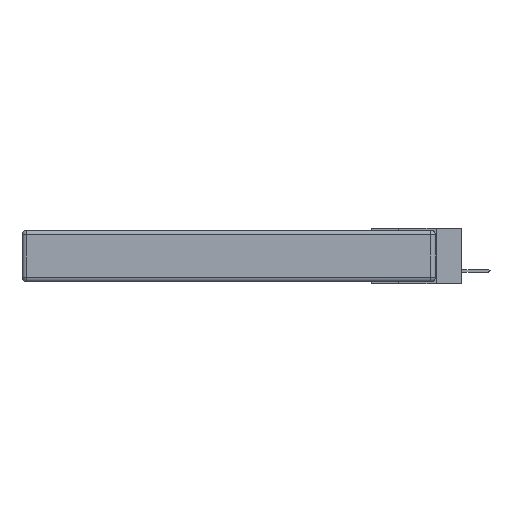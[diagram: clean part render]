
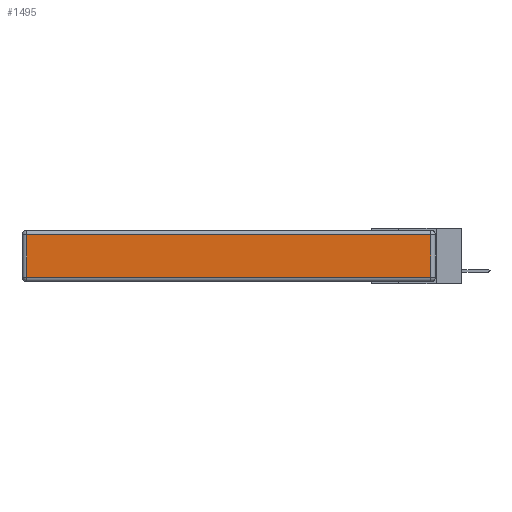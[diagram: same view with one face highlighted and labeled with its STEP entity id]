
A CAD part, left-side view. The second image highlights one B-rep face of the part: STEP entity #1495.
In plain terms, the highlighted planar face has unit normal (-1, 0, 0).
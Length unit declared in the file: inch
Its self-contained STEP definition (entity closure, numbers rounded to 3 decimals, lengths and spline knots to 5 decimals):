
#740 = CARTESIAN_POINT ( 'NONE',  ( 0., 0., -0.343 ) ) ;
#881 = VECTOR ( 'NONE', #3695, 39.37008 ) ;
#1281 = CARTESIAN_POINT ( 'NONE',  ( 0., 2.72, -0.313 ) ) ;
#1439 = CARTESIAN_POINT ( 'NONE',  ( 0., 2.75, -0.03 ) ) ;
#1495 = ADVANCED_FACE ( 'NONE', ( #2724 ), #4963, .T. ) ;
#2037 = DIRECTION ( 'NONE',  ( 0., -1., 0. ) ) ;
#2084 = EDGE_LOOP ( 'NONE', ( #7921, #6473, #15556, #9014 ) ) ;
#2553 = VERTEX_POINT ( 'NONE', #11875 ) ;
#2724 = FACE_OUTER_BOUND ( 'NONE', #2084, .T. ) ;
#3279 = AXIS2_PLACEMENT_3D ( 'NONE', #740, #6346, #15831 ) ;
#3695 = DIRECTION ( 'NONE',  ( 0., 0., -1. ) ) ;
#4009 = VERTEX_POINT ( 'NONE', #14608 ) ;
#4153 = DIRECTION ( 'NONE',  ( 0., 1., 0. ) ) ;
#4963 = PLANE ( 'NONE',  #3279 ) ;
#5562 = VERTEX_POINT ( 'NONE', #1281 ) ;
#6346 = DIRECTION ( 'NONE',  ( -1., 0., 0. ) ) ;
#6473 = ORIENTED_EDGE ( 'NONE', *, *, #13235, .T. ) ;
#6978 = LINE ( 'NONE', #15562, #14504 ) ;
#7324 = EDGE_CURVE ( 'NONE', #4009, #5562, #16681, .T. ) ;
#7921 = ORIENTED_EDGE ( 'NONE', *, *, #17411, .T. ) ;
#8773 = DIRECTION ( 'NONE',  ( 0., 0., 1. ) ) ;
#9014 = ORIENTED_EDGE ( 'NONE', *, *, #7324, .T. ) ;
#11772 = CARTESIAN_POINT ( 'NONE',  ( 0., 2.72, -0.343 ) ) ;
#11875 = CARTESIAN_POINT ( 'NONE',  ( 0., 0.03, -0.313 ) ) ;
#12339 = EDGE_CURVE ( 'NONE', #17239, #4009, #16333, .T. ) ;
#13235 = EDGE_CURVE ( 'NONE', #2553, #17239, #14601, .T. ) ;
#13910 = CARTESIAN_POINT ( 'NONE',  ( 0., 0.03, -0.03 ) ) ;
#14409 = VECTOR ( 'NONE', #4153, 39.37008 ) ;
#14504 = VECTOR ( 'NONE', #2037, 39.37008 ) ;
#14601 = LINE ( 'NONE', #15453, #16087 ) ;
#14608 = CARTESIAN_POINT ( 'NONE',  ( 0., 2.72, -0.03 ) ) ;
#15453 = CARTESIAN_POINT ( 'NONE',  ( 0., 0.03, -0.343 ) ) ;
#15556 = ORIENTED_EDGE ( 'NONE', *, *, #12339, .T. ) ;
#15562 = CARTESIAN_POINT ( 'NONE',  ( 0., 0., -0.313 ) ) ;
#15831 = DIRECTION ( 'NONE',  ( 0., 0., 1. ) ) ;
#16087 = VECTOR ( 'NONE', #8773, 39.37008 ) ;
#16333 = LINE ( 'NONE', #1439, #14409 ) ;
#16681 = LINE ( 'NONE', #11772, #881 ) ;
#17239 = VERTEX_POINT ( 'NONE', #13910 ) ;
#17411 = EDGE_CURVE ( 'NONE', #5562, #2553, #6978, .T. ) ;
